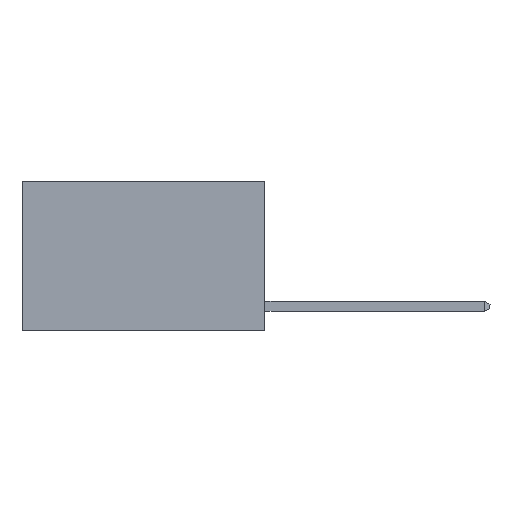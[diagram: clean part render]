
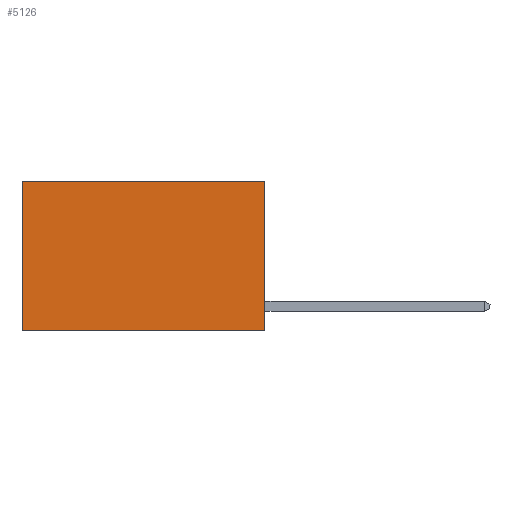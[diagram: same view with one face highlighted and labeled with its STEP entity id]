
A CAD part, left-side view. The second image highlights one B-rep face of the part: STEP entity #5126.
In plain terms, the highlighted planar face has unit normal (-1, 0, 0).
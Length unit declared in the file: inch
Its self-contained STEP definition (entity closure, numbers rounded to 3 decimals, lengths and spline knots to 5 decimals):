
#39 = VERTEX_POINT ( 'NONE', #5206 ) ;
#54 = ORIENTED_EDGE ( 'NONE', *, *, #7528, .T. ) ;
#322 = CARTESIAN_POINT ( 'NONE',  ( 0.2625, 0., 0. ) ) ;
#763 = VERTEX_POINT ( 'NONE', #7151 ) ;
#799 = EDGE_CURVE ( 'NONE', #5761, #763, #2469, .T. ) ;
#1503 = LINE ( 'NONE', #12809, #12830 ) ;
#2021 = EDGE_LOOP ( 'NONE', ( #54, #8385, #9803, #2539 ) ) ;
#2414 = DIRECTION ( 'NONE',  ( 0., 0., -1. ) ) ;
#2469 = LINE ( 'NONE', #10711, #4934 ) ;
#2539 = ORIENTED_EDGE ( 'NONE', *, *, #799, .T. ) ;
#2927 = DIRECTION ( 'NONE',  ( 0., 1., 0. ) ) ;
#4086 = VERTEX_POINT ( 'NONE', #5452 ) ;
#4310 = DIRECTION ( 'NONE',  ( 1., 0., 0. ) ) ;
#4556 = FACE_OUTER_BOUND ( 'NONE', #2021, .T. ) ;
#4934 = VECTOR ( 'NONE', #7416, 39.37008 ) ;
#5126 = ADVANCED_FACE ( 'NONE', ( #4556 ), #9248, .F. ) ;
#5206 = CARTESIAN_POINT ( 'NONE',  ( 0.2625, 0.6, -0.37 ) ) ;
#5452 = CARTESIAN_POINT ( 'NONE',  ( 0.2625, 0., -0.37 ) ) ;
#5637 = VECTOR ( 'NONE', #2414, 39.37008 ) ;
#5761 = VERTEX_POINT ( 'NONE', #322 ) ;
#6346 = CARTESIAN_POINT ( 'NONE',  ( 0.2625, 0., 0. ) ) ;
#7101 = EDGE_CURVE ( 'NONE', #4086, #39, #1503, .T. ) ;
#7151 = CARTESIAN_POINT ( 'NONE',  ( 0.2625, 0.6, 0. ) ) ;
#7416 = DIRECTION ( 'NONE',  ( 0., 1., 0. ) ) ;
#7528 = EDGE_CURVE ( 'NONE', #763, #39, #13121, .T. ) ;
#7670 = VECTOR ( 'NONE', #13128, 39.37008 ) ;
#8092 = EDGE_CURVE ( 'NONE', #5761, #4086, #13108, .T. ) ;
#8385 = ORIENTED_EDGE ( 'NONE', *, *, #7101, .F. ) ;
#9248 = PLANE ( 'NONE',  #9441 ) ;
#9273 = CARTESIAN_POINT ( 'NONE',  ( 0.2625, 0., 0. ) ) ;
#9441 = AXIS2_PLACEMENT_3D ( 'NONE', #6346, #4310, #11193 ) ;
#9803 = ORIENTED_EDGE ( 'NONE', *, *, #8092, .F. ) ;
#10438 = CARTESIAN_POINT ( 'NONE',  ( 0.2625, 0.6, 0. ) ) ;
#10711 = CARTESIAN_POINT ( 'NONE',  ( 0.2625, 0., 0. ) ) ;
#11193 = DIRECTION ( 'NONE',  ( 0., 0., -1. ) ) ;
#12809 = CARTESIAN_POINT ( 'NONE',  ( 0.2625, 0., -0.37 ) ) ;
#12830 = VECTOR ( 'NONE', #2927, 39.37008 ) ;
#13108 = LINE ( 'NONE', #9273, #7670 ) ;
#13121 = LINE ( 'NONE', #10438, #5637 ) ;
#13128 = DIRECTION ( 'NONE',  ( 0., 0., -1. ) ) ;
